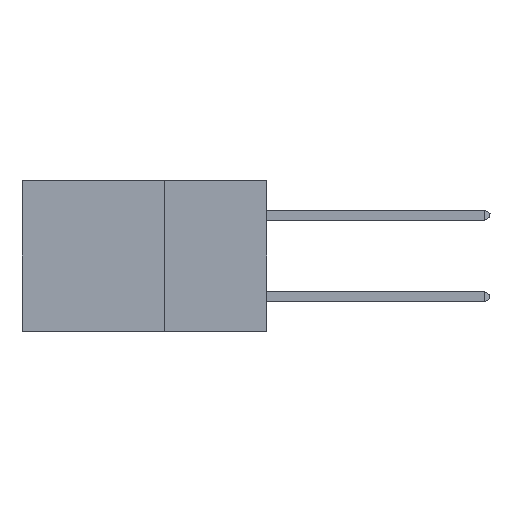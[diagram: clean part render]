
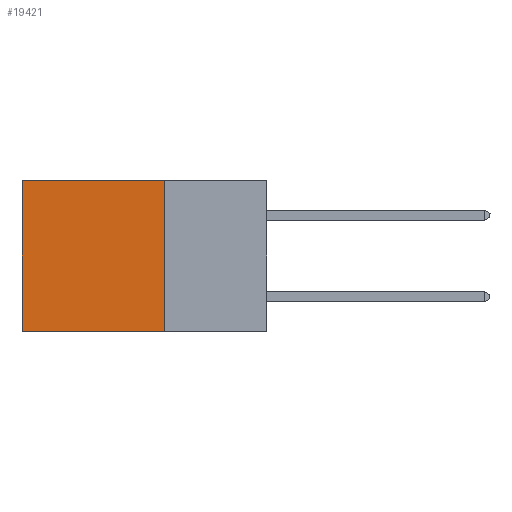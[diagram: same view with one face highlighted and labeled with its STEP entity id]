
A CAD part, left-side view. The second image highlights one B-rep face of the part: STEP entity #19421.
In plain terms, the highlighted planar face has unit normal (-1, 0, 0).
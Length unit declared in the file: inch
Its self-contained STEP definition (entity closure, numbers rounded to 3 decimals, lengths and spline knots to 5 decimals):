
#317 = LINE ( 'NONE', #20766, #20345 ) ;
#692 = ORIENTED_EDGE ( 'NONE', *, *, #14363, .T. ) ;
#997 = ORIENTED_EDGE ( 'NONE', *, *, #14007, .F. ) ;
#1468 = CARTESIAN_POINT ( 'NONE',  ( 0.2875, 0.6, 0. ) ) ;
#2059 = VECTOR ( 'NONE', #13106, 39.37008 ) ;
#2263 = PLANE ( 'NONE',  #5631 ) ;
#2475 = EDGE_CURVE ( 'NONE', #2495, #17892, #11590, .T. ) ;
#2495 = VERTEX_POINT ( 'NONE', #13633 ) ;
#3987 = CARTESIAN_POINT ( 'NONE',  ( 0.2875, 0.6, 0. ) ) ;
#5631 = AXIS2_PLACEMENT_3D ( 'NONE', #9597, #9837, #15217 ) ;
#5644 = FACE_OUTER_BOUND ( 'NONE', #9813, .T. ) ;
#5779 = EDGE_CURVE ( 'NONE', #18754, #9301, #21385, .T. ) ;
#7104 = ORIENTED_EDGE ( 'NONE', *, *, #2475, .F. ) ;
#9301 = VERTEX_POINT ( 'NONE', #15007 ) ;
#9597 = CARTESIAN_POINT ( 'NONE',  ( 0.2875, 0.25, 0. ) ) ;
#9813 = EDGE_LOOP ( 'NONE', ( #23359, #997, #7104, #692 ) ) ;
#9837 = DIRECTION ( 'NONE',  ( 1., 0., 0. ) ) ;
#9937 = CARTESIAN_POINT ( 'NONE',  ( 0.2875, 0.25, -0.37 ) ) ;
#11225 = DIRECTION ( 'NONE',  ( 0., 1., 0. ) ) ;
#11590 = LINE ( 'NONE', #13157, #13131 ) ;
#11710 = DIRECTION ( 'NONE',  ( 0., 0., -1. ) ) ;
#13106 = DIRECTION ( 'NONE',  ( 0., 0., -1. ) ) ;
#13131 = VECTOR ( 'NONE', #11710, 39.37008 ) ;
#13157 = CARTESIAN_POINT ( 'NONE',  ( 0.2875, 0.25, 0. ) ) ;
#13633 = CARTESIAN_POINT ( 'NONE',  ( 0.2875, 0.25, 0. ) ) ;
#14007 = EDGE_CURVE ( 'NONE', #17892, #9301, #20700, .T. ) ;
#14363 = EDGE_CURVE ( 'NONE', #2495, #18754, #317, .T. ) ;
#14950 = CARTESIAN_POINT ( 'NONE',  ( 0.2875, 0.25, -0.37 ) ) ;
#15007 = CARTESIAN_POINT ( 'NONE',  ( 0.2875, 0.6, -0.37 ) ) ;
#15217 = DIRECTION ( 'NONE',  ( 0., 0., -1. ) ) ;
#17892 = VERTEX_POINT ( 'NONE', #14950 ) ;
#18754 = VERTEX_POINT ( 'NONE', #1468 ) ;
#19002 = VECTOR ( 'NONE', #19384, 39.37008 ) ;
#19384 = DIRECTION ( 'NONE',  ( 0., 1., 0. ) ) ;
#19421 = ADVANCED_FACE ( 'NONE', ( #5644 ), #2263, .F. ) ;
#20345 = VECTOR ( 'NONE', #11225, 39.37008 ) ;
#20700 = LINE ( 'NONE', #9937, #19002 ) ;
#20766 = CARTESIAN_POINT ( 'NONE',  ( 0.2875, 0.25, 0. ) ) ;
#21385 = LINE ( 'NONE', #3987, #2059 ) ;
#23359 = ORIENTED_EDGE ( 'NONE', *, *, #5779, .T. ) ;
